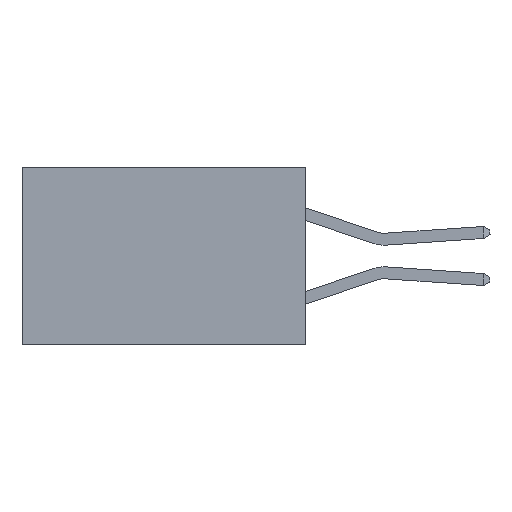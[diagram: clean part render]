
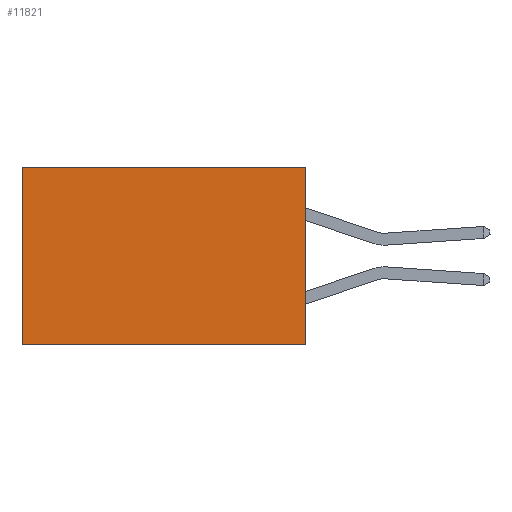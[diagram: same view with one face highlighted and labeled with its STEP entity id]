
A CAD part, left-side view. The second image highlights one B-rep face of the part: STEP entity #11821.
In plain terms, the highlighted planar face has unit normal (-1, 0, 0).
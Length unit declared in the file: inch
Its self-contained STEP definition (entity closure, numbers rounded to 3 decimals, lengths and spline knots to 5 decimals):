
#216 = EDGE_CURVE ( 'NONE', #12543, #9856, #16618, .T. ) ;
#285 = LINE ( 'NONE', #1154, #4005 ) ;
#329 = DIRECTION ( 'NONE',  ( 0., 1., 0. ) ) ;
#1154 = CARTESIAN_POINT ( 'NONE',  ( 0.277, 0., -0.37 ) ) ;
#1413 = EDGE_LOOP ( 'NONE', ( #8793, #10059, #13956, #10874 ) ) ;
#2567 = DIRECTION ( 'NONE',  ( 0., 1., 0. ) ) ;
#2658 = CARTESIAN_POINT ( 'NONE',  ( 0.277, 0., -0.37 ) ) ;
#4005 = VECTOR ( 'NONE', #2567, 39.37008 ) ;
#4518 = VERTEX_POINT ( 'NONE', #7593 ) ;
#4693 = LINE ( 'NONE', #2658, #14527 ) ;
#5246 = DIRECTION ( 'NONE',  ( 1., 0., 0. ) ) ;
#6387 = FACE_OUTER_BOUND ( 'NONE', #1413, .T. ) ;
#7045 = DIRECTION ( 'NONE',  ( 0., 0., -1. ) ) ;
#7053 = CARTESIAN_POINT ( 'NONE',  ( 0.277, 0., -0.37 ) ) ;
#7593 = CARTESIAN_POINT ( 'NONE',  ( 0.277, 0.59, -0.37 ) ) ;
#7630 = VERTEX_POINT ( 'NONE', #7053 ) ;
#8793 = ORIENTED_EDGE ( 'NONE', *, *, #10778, .T. ) ;
#9208 = CARTESIAN_POINT ( 'NONE',  ( 0.277, 0.59, 0. ) ) ;
#9264 = PLANE ( 'NONE',  #16036 ) ;
#9368 = LINE ( 'NONE', #13629, #15962 ) ;
#9856 = VERTEX_POINT ( 'NONE', #9208 ) ;
#10059 = ORIENTED_EDGE ( 'NONE', *, *, #11302, .F. ) ;
#10678 = EDGE_CURVE ( 'NONE', #12543, #7630, #4693, .T. ) ;
#10778 = EDGE_CURVE ( 'NONE', #9856, #4518, #9368, .T. ) ;
#10874 = ORIENTED_EDGE ( 'NONE', *, *, #216, .T. ) ;
#11302 = EDGE_CURVE ( 'NONE', #7630, #4518, #285, .T. ) ;
#11821 = ADVANCED_FACE ( 'NONE', ( #6387 ), #9264, .F. ) ;
#12203 = CARTESIAN_POINT ( 'NONE',  ( 0.277, 0., 0. ) ) ;
#12543 = VERTEX_POINT ( 'NONE', #12203 ) ;
#13128 = VECTOR ( 'NONE', #329, 39.37008 ) ;
#13466 = DIRECTION ( 'NONE',  ( 0., 0., -1. ) ) ;
#13629 = CARTESIAN_POINT ( 'NONE',  ( 0.277, 0.59, -0.37 ) ) ;
#13956 = ORIENTED_EDGE ( 'NONE', *, *, #10678, .F. ) ;
#14527 = VECTOR ( 'NONE', #13466, 39.37008 ) ;
#14580 = DIRECTION ( 'NONE',  ( 0., 0., -1. ) ) ;
#14701 = CARTESIAN_POINT ( 'NONE',  ( 0.277, 0., 0. ) ) ;
#15962 = VECTOR ( 'NONE', #7045, 39.37008 ) ;
#16036 = AXIS2_PLACEMENT_3D ( 'NONE', #17184, #5246, #14580 ) ;
#16618 = LINE ( 'NONE', #14701, #13128 ) ;
#17184 = CARTESIAN_POINT ( 'NONE',  ( 0.277, 0., -0.37 ) ) ;
